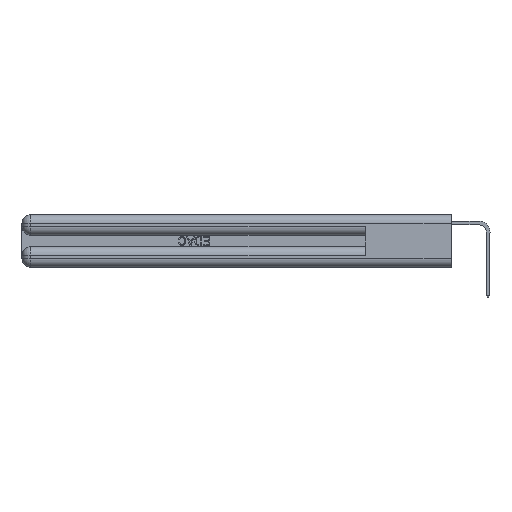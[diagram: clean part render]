
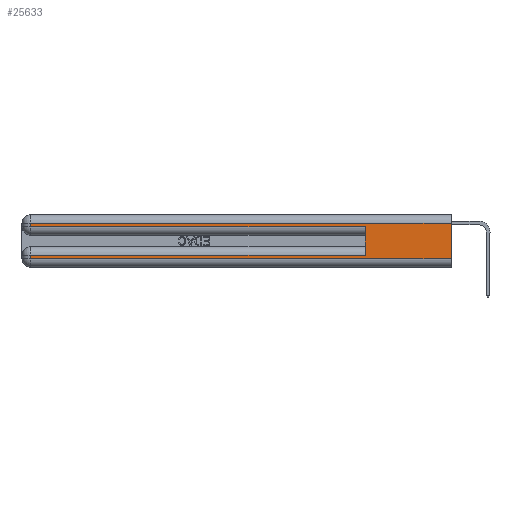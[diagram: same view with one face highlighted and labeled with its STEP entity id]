
A CAD part, left-side view. The second image highlights one B-rep face of the part: STEP entity #25633.
In plain terms, the highlighted planar face has unit normal (-1, 0, 0).
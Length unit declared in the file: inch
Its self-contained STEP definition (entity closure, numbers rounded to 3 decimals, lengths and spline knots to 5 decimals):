
#147 = ORIENTED_EDGE ( 'NONE', *, *, #25462, .F. ) ;
#682 = PLANE ( 'NONE',  #7900 ) ;
#1000 = VERTEX_POINT ( 'NONE', #10269 ) ;
#1248 = VECTOR ( 'NONE', #15051, 39.37008 ) ;
#1396 = CARTESIAN_POINT ( 'NONE',  ( 0., 2.94, 0.285 ) ) ;
#1517 = DIRECTION ( 'NONE',  ( 0., 0., -1. ) ) ;
#2223 = CARTESIAN_POINT ( 'NONE',  ( 0., 0., 0.37 ) ) ;
#2507 = CARTESIAN_POINT ( 'NONE',  ( 0., 0., 0.06 ) ) ;
#2573 = CARTESIAN_POINT ( 'NONE',  ( 0., 0.6, 0.145 ) ) ;
#2629 = VERTEX_POINT ( 'NONE', #22706 ) ;
#2764 = VECTOR ( 'NONE', #23538, 39.37008 ) ;
#3203 = ORIENTED_EDGE ( 'NONE', *, *, #7290, .T. ) ;
#3330 = CARTESIAN_POINT ( 'NONE',  ( 0., 0.6, 0.085 ) ) ;
#4671 = DIRECTION ( 'NONE',  ( 0., 0., 1. ) ) ;
#4932 = DIRECTION ( 'NONE',  ( 0., 0., -1. ) ) ;
#5320 = ORIENTED_EDGE ( 'NONE', *, *, #17278, .T. ) ;
#5474 = ORIENTED_EDGE ( 'NONE', *, *, #21470, .T. ) ;
#5763 = ORIENTED_EDGE ( 'NONE', *, *, #14828, .T. ) ;
#6427 = EDGE_CURVE ( 'NONE', #26285, #2629, #22176, .T. ) ;
#7290 = EDGE_CURVE ( 'NONE', #15367, #24639, #12982, .T. ) ;
#7782 = LINE ( 'NONE', #26444, #18274 ) ;
#7900 = AXIS2_PLACEMENT_3D ( 'NONE', #13246, #17467, #4932 ) ;
#8086 = VERTEX_POINT ( 'NONE', #3330 ) ;
#8739 = CARTESIAN_POINT ( 'NONE',  ( 0., 0., 0.31 ) ) ;
#9073 = VECTOR ( 'NONE', #17377, 39.37008 ) ;
#9808 = CARTESIAN_POINT ( 'NONE',  ( 0., 2.94, 0.31 ) ) ;
#10241 = CARTESIAN_POINT ( 'NONE',  ( 0., 0., 0.285 ) ) ;
#10269 = CARTESIAN_POINT ( 'NONE',  ( 0., 2.94, 0.06 ) ) ;
#12982 = LINE ( 'NONE', #8739, #1248 ) ;
#13064 = EDGE_CURVE ( 'NONE', #1000, #25003, #13868, .T. ) ;
#13142 = VERTEX_POINT ( 'NONE', #23806 ) ;
#13246 = CARTESIAN_POINT ( 'NONE',  ( 0., 0., 0.37 ) ) ;
#13868 = LINE ( 'NONE', #21481, #2764 ) ;
#14517 = VECTOR ( 'NONE', #4671, 39.37008 ) ;
#14828 = EDGE_CURVE ( 'NONE', #24639, #26285, #21299, .T. ) ;
#15051 = DIRECTION ( 'NONE',  ( 0., 1., 0. ) ) ;
#15072 = VECTOR ( 'NONE', #22508, 39.37008 ) ;
#15367 = VERTEX_POINT ( 'NONE', #21951 ) ;
#16241 = CARTESIAN_POINT ( 'NONE',  ( 0., 2.94, 0.37 ) ) ;
#16459 = VECTOR ( 'NONE', #16840, 39.37008 ) ;
#16628 = VECTOR ( 'NONE', #26894, 39.37008 ) ;
#16840 = DIRECTION ( 'NONE',  ( 0., 0., -1. ) ) ;
#17118 = LINE ( 'NONE', #2223, #16459 ) ;
#17278 = EDGE_CURVE ( 'NONE', #13142, #1000, #7782, .T. ) ;
#17377 = DIRECTION ( 'NONE',  ( 0., 1., 0. ) ) ;
#17467 = DIRECTION ( 'NONE',  ( 1., 0., 0. ) ) ;
#18274 = VECTOR ( 'NONE', #1517, 39.37008 ) ;
#18757 = FACE_OUTER_BOUND ( 'NONE', #21174, .T. ) ;
#20741 = LINE ( 'NONE', #2573, #14517 ) ;
#20834 = ORIENTED_EDGE ( 'NONE', *, *, #23711, .F. ) ;
#21174 = EDGE_LOOP ( 'NONE', ( #147, #3203, #5763, #26198, #20834, #5474, #5320, #23676 ) ) ;
#21299 = LINE ( 'NONE', #16241, #15072 ) ;
#21470 = EDGE_CURVE ( 'NONE', #8086, #13142, #25058, .T. ) ;
#21481 = CARTESIAN_POINT ( 'NONE',  ( 0., 0., 0.06 ) ) ;
#21951 = CARTESIAN_POINT ( 'NONE',  ( 0., 0., 0.31 ) ) ;
#22176 = LINE ( 'NONE', #10241, #16628 ) ;
#22508 = DIRECTION ( 'NONE',  ( 0., 0., -1. ) ) ;
#22706 = CARTESIAN_POINT ( 'NONE',  ( 0., 0.6, 0.285 ) ) ;
#23538 = DIRECTION ( 'NONE',  ( 0., -1., 0. ) ) ;
#23542 = CARTESIAN_POINT ( 'NONE',  ( 0., 0., 0.085 ) ) ;
#23676 = ORIENTED_EDGE ( 'NONE', *, *, #13064, .T. ) ;
#23711 = EDGE_CURVE ( 'NONE', #8086, #2629, #20741, .T. ) ;
#23806 = CARTESIAN_POINT ( 'NONE',  ( 0., 2.94, 0.085 ) ) ;
#24639 = VERTEX_POINT ( 'NONE', #9808 ) ;
#25003 = VERTEX_POINT ( 'NONE', #2507 ) ;
#25058 = LINE ( 'NONE', #23542, #9073 ) ;
#25462 = EDGE_CURVE ( 'NONE', #15367, #25003, #17118, .T. ) ;
#25633 = ADVANCED_FACE ( 'NONE', ( #18757 ), #682, .F. ) ;
#26198 = ORIENTED_EDGE ( 'NONE', *, *, #6427, .T. ) ;
#26285 = VERTEX_POINT ( 'NONE', #1396 ) ;
#26444 = CARTESIAN_POINT ( 'NONE',  ( 0., 2.94, 0.37 ) ) ;
#26894 = DIRECTION ( 'NONE',  ( 0., -1., 0. ) ) ;
